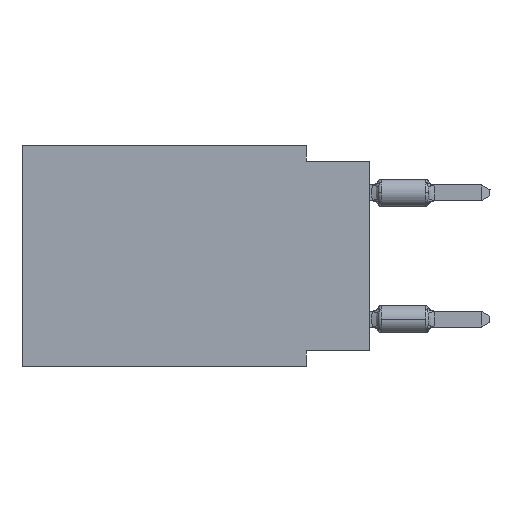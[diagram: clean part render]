
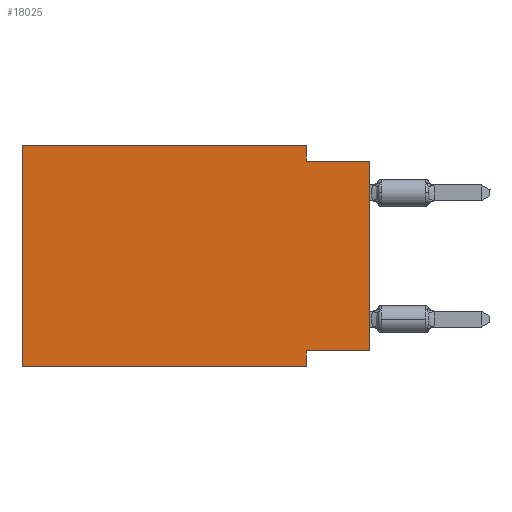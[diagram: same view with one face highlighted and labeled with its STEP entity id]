
A CAD part, left-side view. The second image highlights one B-rep face of the part: STEP entity #18025.
In plain terms, the highlighted planar face has unit normal (-1, 0, 0).
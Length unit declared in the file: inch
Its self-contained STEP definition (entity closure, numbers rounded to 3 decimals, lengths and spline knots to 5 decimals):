
#229 = DIRECTION ( 'NONE',  ( 0., 0., 1. ) ) ;
#1053 = LINE ( 'NONE', #9215, #11431 ) ;
#1757 = CARTESIAN_POINT ( 'NONE',  ( 0., 0.1, -0.025 ) ) ;
#1768 = DIRECTION ( 'NONE',  ( 1., 0., 0. ) ) ;
#2322 = EDGE_CURVE ( 'NONE', #32569, #32864, #14209, .T. ) ;
#3562 = VECTOR ( 'NONE', #27635, 39.37008 ) ;
#5851 = CARTESIAN_POINT ( 'NONE',  ( 0., 0.1, 0. ) ) ;
#5900 = CARTESIAN_POINT ( 'NONE',  ( 0., 0.1, -0.35 ) ) ;
#6280 = LINE ( 'NONE', #22116, #3562 ) ;
#6604 = DIRECTION ( 'NONE',  ( 0., 0., -1. ) ) ;
#7088 = VERTEX_POINT ( 'NONE', #5851 ) ;
#7134 = CARTESIAN_POINT ( 'NONE',  ( 0., 0., -0.025 ) ) ;
#7275 = PLANE ( 'NONE',  #25107 ) ;
#8196 = DIRECTION ( 'NONE',  ( 0., 0., -1. ) ) ;
#9047 = DIRECTION ( 'NONE',  ( 0., 1., 0. ) ) ;
#9215 = CARTESIAN_POINT ( 'NONE',  ( 0., 0.55, -0.35 ) ) ;
#10423 = CARTESIAN_POINT ( 'NONE',  ( 0., 0.55, 0. ) ) ;
#10994 = VECTOR ( 'NONE', #27323, 39.37008 ) ;
#11149 = ORIENTED_EDGE ( 'NONE', *, *, #33625, .F. ) ;
#11396 = CARTESIAN_POINT ( 'NONE',  ( 0., 0., 0. ) ) ;
#11431 = VECTOR ( 'NONE', #28078, 39.37008 ) ;
#11762 = LINE ( 'NONE', #25093, #15827 ) ;
#12114 = VECTOR ( 'NONE', #8196, 39.37008 ) ;
#12129 = CARTESIAN_POINT ( 'NONE',  ( 0., 0.1, -0.325 ) ) ;
#13038 = ORIENTED_EDGE ( 'NONE', *, *, #34013, .T. ) ;
#14209 = LINE ( 'NONE', #32878, #12114 ) ;
#15554 = LINE ( 'NONE', #26402, #27915 ) ;
#15827 = VECTOR ( 'NONE', #6604, 39.37008 ) ;
#16227 = ORIENTED_EDGE ( 'NONE', *, *, #31089, .F. ) ;
#16319 = ORIENTED_EDGE ( 'NONE', *, *, #25092, .F. ) ;
#17109 = ORIENTED_EDGE ( 'NONE', *, *, #19016, .F. ) ;
#17371 = ORIENTED_EDGE ( 'NONE', *, *, #24608, .F. ) ;
#18025 = ADVANCED_FACE ( 'NONE', ( #31623 ), #7275, .F. ) ;
#19016 = EDGE_CURVE ( 'NONE', #23908, #7088, #19164, .T. ) ;
#19081 = LINE ( 'NONE', #11396, #29145 ) ;
#19164 = LINE ( 'NONE', #33191, #10994 ) ;
#20078 = LINE ( 'NONE', #33398, #31157 ) ;
#21279 = ORIENTED_EDGE ( 'NONE', *, *, #30500, .T. ) ;
#22116 = CARTESIAN_POINT ( 'NONE',  ( 0., 0.55, 0. ) ) ;
#23449 = CARTESIAN_POINT ( 'NONE',  ( 0., 0.55, -0.35 ) ) ;
#23908 = VERTEX_POINT ( 'NONE', #10423 ) ;
#24608 = EDGE_CURVE ( 'NONE', #7088, #25268, #11762, .T. ) ;
#25092 = EDGE_CURVE ( 'NONE', #34107, #32569, #20078, .T. ) ;
#25093 = CARTESIAN_POINT ( 'NONE',  ( 0., 0.1, 0. ) ) ;
#25107 = AXIS2_PLACEMENT_3D ( 'NONE', #31795, #1768, #26480 ) ;
#25268 = VERTEX_POINT ( 'NONE', #1757 ) ;
#25276 = VERTEX_POINT ( 'NONE', #23449 ) ;
#26402 = CARTESIAN_POINT ( 'NONE',  ( 0., 0., -0.025 ) ) ;
#26480 = DIRECTION ( 'NONE',  ( 0., 0., -1. ) ) ;
#27274 = ORIENTED_EDGE ( 'NONE', *, *, #2322, .F. ) ;
#27323 = DIRECTION ( 'NONE',  ( 0., -1., 0. ) ) ;
#27635 = DIRECTION ( 'NONE',  ( 0., 0., 1. ) ) ;
#27915 = VECTOR ( 'NONE', #34718, 39.37008 ) ;
#28078 = DIRECTION ( 'NONE',  ( 0., -1., 0. ) ) ;
#29145 = VECTOR ( 'NONE', #229, 39.37008 ) ;
#29401 = EDGE_LOOP ( 'NONE', ( #13038, #16227, #17371, #17109, #11149, #21279, #27274, #16319 ) ) ;
#30500 = EDGE_CURVE ( 'NONE', #25276, #32864, #1053, .T. ) ;
#30582 = CARTESIAN_POINT ( 'NONE',  ( 0., 0., -0.325 ) ) ;
#31089 = EDGE_CURVE ( 'NONE', #25268, #34426, #15554, .T. ) ;
#31157 = VECTOR ( 'NONE', #9047, 39.37008 ) ;
#31623 = FACE_OUTER_BOUND ( 'NONE', #29401, .T. ) ;
#31795 = CARTESIAN_POINT ( 'NONE',  ( 0., 0.55, 0. ) ) ;
#32569 = VERTEX_POINT ( 'NONE', #12129 ) ;
#32864 = VERTEX_POINT ( 'NONE', #5900 ) ;
#32878 = CARTESIAN_POINT ( 'NONE',  ( 0., 0.1, -0.35 ) ) ;
#33191 = CARTESIAN_POINT ( 'NONE',  ( 0., 0.55, 0. ) ) ;
#33398 = CARTESIAN_POINT ( 'NONE',  ( 0., 0., -0.325 ) ) ;
#33625 = EDGE_CURVE ( 'NONE', #25276, #23908, #6280, .T. ) ;
#34013 = EDGE_CURVE ( 'NONE', #34107, #34426, #19081, .T. ) ;
#34107 = VERTEX_POINT ( 'NONE', #30582 ) ;
#34426 = VERTEX_POINT ( 'NONE', #7134 ) ;
#34718 = DIRECTION ( 'NONE',  ( 0., -1., 0. ) ) ;
